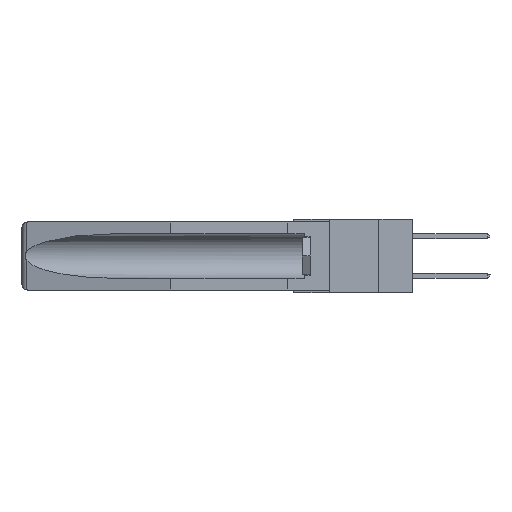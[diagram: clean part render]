
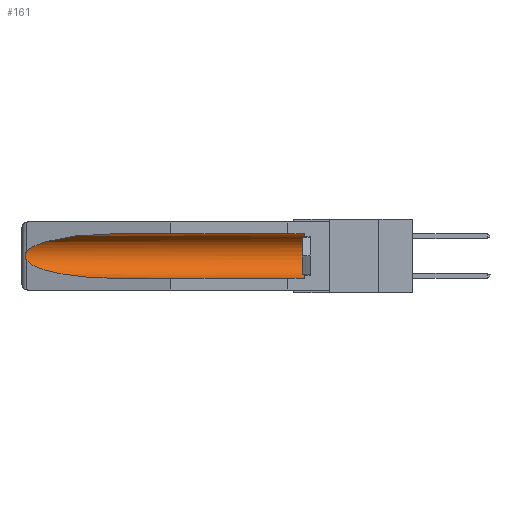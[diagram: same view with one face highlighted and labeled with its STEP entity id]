
A CAD part, left-side view. The second image highlights one B-rep face of the part: STEP entity #161.
In plain terms, the highlighted cylindrical face has radius 2.857 mm (diameter 5.715 mm), a partial arc.
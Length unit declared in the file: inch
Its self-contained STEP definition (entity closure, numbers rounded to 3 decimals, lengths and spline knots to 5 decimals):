
#28 = CARTESIAN_POINT ( 'NONE',  ( 0.155, 1.07973, -0.284 ) ) ;
#161 = ADVANCED_FACE ( 'NONE', ( #2619 ), #9265, .F. ) ;
#649 = EDGE_CURVE ( 'NONE', #16193, #15824, #2980, .T. ) ;
#2229 = VERTEX_POINT ( 'NONE', #28 ) ;
#2322 = CARTESIAN_POINT ( 'NONE',  ( 0.26655, 1.53094, -0.18657 ) ) ;
#2442 = CARTESIAN_POINT ( 'NONE',  ( 0.2673, 1.53269, -0.17917 ) ) ;
#2619 = FACE_OUTER_BOUND ( 'NONE', #12529, .T. ) ;
#2640 = ORIENTED_EDGE ( 'NONE', *, *, #649, .T. ) ;
#2740 = CARTESIAN_POINT ( 'NONE',  ( 0.21114, 1.30732, -0.059 ) ) ;
#2842 = EDGE_CURVE ( 'NONE', #16306, #2229, #16345, .T. ) ;
#2980 = LINE ( 'NONE', #11606, #14570 ) ;
#3374 = AXIS2_PLACEMENT_3D ( 'NONE', #16275, #8413, #4554 ) ;
#3498 = CARTESIAN_POINT ( 'NONE',  ( 0.155, -0.30754, -0.284 ) ) ;
#3607 = CARTESIAN_POINT ( 'NONE',  ( 0.25451, 1.48313, -0.24835 ) ) ;
#4153 =( BOUNDED_CURVE ( )  B_SPLINE_CURVE ( 3, ( #12234, #3607, #12977, #12737 ),
 .UNSPECIFIED., .F., .F. ) 
 B_SPLINE_CURVE_WITH_KNOTS ( ( 4, 4 ),
 ( 0.1948, 1.5708 ),
 .UNSPECIFIED. ) 
 CURVE ( )  GEOMETRIC_REPRESENTATION_ITEM ( )  RATIONAL_B_SPLINE_CURVE ( ( 1., 0.848, 0.848, 1. ) ) 
 REPRESENTATION_ITEM ( '' )  );
#4238 = ORIENTED_EDGE ( 'NONE', *, *, #12294, .T. ) ;
#4554 = DIRECTION ( 'NONE',  ( 0., 0., 1. ) ) ;
#4730 = CIRCLE ( 'NONE', #3374, 0.1125 ) ;
#4925 = DIRECTION ( 'NONE',  ( 0., 1., 0. ) ) ;
#4938 = CARTESIAN_POINT ( 'NONE',  ( 0.26537, 1.52718, -0.14972 ) ) ;
#5161 = CARTESIAN_POINT ( 'NONE',  ( 0.155, 1.07973, -0.059 ) ) ;
#5289 = CARTESIAN_POINT ( 'NONE',  ( 0.26537, 1.52718, -0.14972 ) ) ;
#5851 = CARTESIAN_POINT ( 'NONE',  ( 0.155, 0.126, -0.059 ) ) ;
#6163 = CARTESIAN_POINT ( 'NONE',  ( 0.26654, 1.53092, -0.15636 ) ) ;
#6206 = DIRECTION ( 'NONE',  ( 0., 0., 1. ) ) ;
#6279 = CARTESIAN_POINT ( 'NONE',  ( 0.2675, 1.53308, -0.16763 ) ) ;
#6582 = ORIENTED_EDGE ( 'NONE', *, *, #2842, .F. ) ;
#6873 = VERTEX_POINT ( 'NONE', #16821 ) ;
#7587 = DIRECTION ( 'NONE',  ( 0., 1., 0. ) ) ;
#7749 = CARTESIAN_POINT ( 'NONE',  ( 0.2675, 1.53308, -0.17534 ) ) ;
#8206 = ORIENTED_EDGE ( 'NONE', *, *, #9407, .T. ) ;
#8413 = DIRECTION ( 'NONE',  ( 0., -1., 0. ) ) ;
#8431 = AXIS2_PLACEMENT_3D ( 'NONE', #10202, #10036, #6206 ) ;
#8835 = CARTESIAN_POINT ( 'NONE',  ( 0.2673, 1.5327, -0.16383 ) ) ;
#9265 = CYLINDRICAL_SURFACE ( 'NONE', #8431, 0.1125 ) ;
#9407 = EDGE_CURVE ( 'NONE', #16306, #16193, #4730, .T. ) ;
#9596 =( BOUNDED_CURVE ( )  B_SPLINE_CURVE ( 3, ( #15729, #2740, #15786, #5289 ),
 .UNSPECIFIED., .F., .F. ) 
 B_SPLINE_CURVE_WITH_KNOTS ( ( 4, 4 ),
 ( 4.71239, 6.08839 ),
 .UNSPECIFIED. ) 
 CURVE ( )  GEOMETRIC_REPRESENTATION_ITEM ( )  RATIONAL_B_SPLINE_CURVE ( ( 1., 0.848, 0.848, 1. ) ) 
 REPRESENTATION_ITEM ( '' )  );
#9978 = VECTOR ( 'NONE', #4925, 39.37008 ) ;
#10036 = DIRECTION ( 'NONE',  ( 0., 1., 0. ) ) ;
#10202 = CARTESIAN_POINT ( 'NONE',  ( 0.155, -0.30754, -0.1715 ) ) ;
#10344 = VERTEX_POINT ( 'NONE', #13220 ) ;
#11264 = ORIENTED_EDGE ( 'NONE', *, *, #13836, .T. ) ;
#11601 = CARTESIAN_POINT ( 'NONE',  ( 0.26597, 1.5296, -0.19026 ) ) ;
#11606 = CARTESIAN_POINT ( 'NONE',  ( 0.155, -0.30754, -0.059 ) ) ;
#11985 = EDGE_CURVE ( 'NONE', #10344, #2229, #4153, .T. ) ;
#12234 = CARTESIAN_POINT ( 'NONE',  ( 0.26537, 1.52718, -0.19328 ) ) ;
#12294 = EDGE_CURVE ( 'NONE', #15824, #6873, #9596, .T. ) ;
#12529 = EDGE_LOOP ( 'NONE', ( #4238, #11264, #15749, #6582, #8206, #2640 ) ) ;
#12737 = CARTESIAN_POINT ( 'NONE',  ( 0.155, 1.07973, -0.284 ) ) ;
#12977 = CARTESIAN_POINT ( 'NONE',  ( 0.21114, 1.30732, -0.284 ) ) ;
#13220 = CARTESIAN_POINT ( 'NONE',  ( 0.26537, 1.52718, -0.19328 ) ) ;
#13836 = EDGE_CURVE ( 'NONE', #6873, #10344, #15170, .T. ) ;
#13957 = CARTESIAN_POINT ( 'NONE',  ( 0.155, 0.126, -0.284 ) ) ;
#14309 = CARTESIAN_POINT ( 'NONE',  ( 0.26597, 1.52961, -0.15275 ) ) ;
#14570 = VECTOR ( 'NONE', #7587, 39.37008 ) ;
#15170 = B_SPLINE_CURVE_WITH_KNOTS ( 'NONE', 3,
 ( #4938, #14309, #6163, #8835, #6279, #7749, #2442, #2322, #11601, #15381 ),
 .UNSPECIFIED., .F., .F.,
 ( 4, 2, 2, 2, 4 ),
 ( 0., 0.00029, 0.00058, 0.00087, 0.00117 ),
 .UNSPECIFIED. ) ;
#15381 = CARTESIAN_POINT ( 'NONE',  ( 0.26537, 1.52718, -0.19328 ) ) ;
#15729 = CARTESIAN_POINT ( 'NONE',  ( 0.155, 1.07973, -0.059 ) ) ;
#15749 = ORIENTED_EDGE ( 'NONE', *, *, #11985, .T. ) ;
#15786 = CARTESIAN_POINT ( 'NONE',  ( 0.25451, 1.48313, -0.09465 ) ) ;
#15824 = VERTEX_POINT ( 'NONE', #5161 ) ;
#16193 = VERTEX_POINT ( 'NONE', #5851 ) ;
#16275 = CARTESIAN_POINT ( 'NONE',  ( 0.155, 0.126, -0.1715 ) ) ;
#16306 = VERTEX_POINT ( 'NONE', #13957 ) ;
#16345 = LINE ( 'NONE', #3498, #9978 ) ;
#16821 = CARTESIAN_POINT ( 'NONE',  ( 0.26537, 1.52718, -0.14972 ) ) ;
